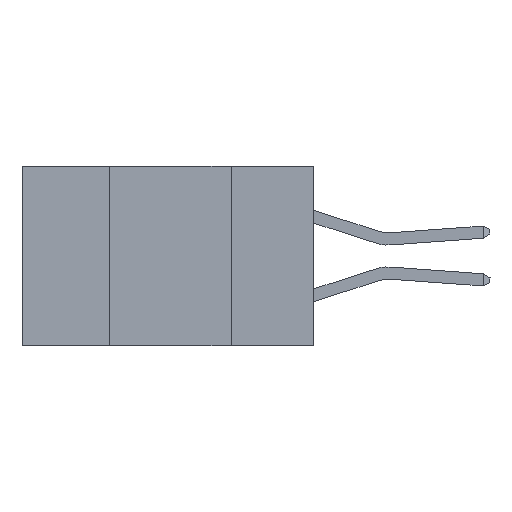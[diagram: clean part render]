
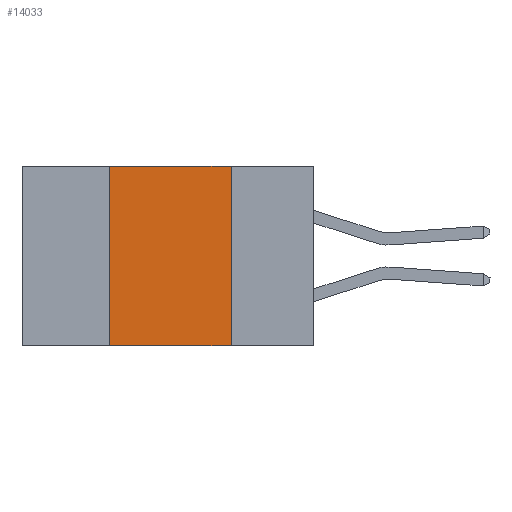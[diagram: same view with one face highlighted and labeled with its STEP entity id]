
A CAD part, left-side view. The second image highlights one B-rep face of the part: STEP entity #14033.
In plain terms, the highlighted planar face has unit normal (-1, 0, 0).
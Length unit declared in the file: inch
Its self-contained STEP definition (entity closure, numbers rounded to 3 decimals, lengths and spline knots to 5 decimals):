
#760 = CARTESIAN_POINT ( 'NONE',  ( 0., 0.17, 0. ) ) ;
#1239 = CARTESIAN_POINT ( 'NONE',  ( 0., 0.42, -0.37 ) ) ;
#2269 = VECTOR ( 'NONE', #9931, 39.37008 ) ;
#2905 = VECTOR ( 'NONE', #11522, 39.37008 ) ;
#3263 = CARTESIAN_POINT ( 'NONE',  ( 0., 0.6, -0.37 ) ) ;
#3797 = EDGE_CURVE ( 'NONE', #12333, #7902, #7656, .T. ) ;
#4444 = ORIENTED_EDGE ( 'NONE', *, *, #6841, .F. ) ;
#4681 = PLANE ( 'NONE',  #9546 ) ;
#4725 = LINE ( 'NONE', #14115, #2269 ) ;
#4855 = DIRECTION ( 'NONE',  ( 0., 0., -1. ) ) ;
#4933 = CARTESIAN_POINT ( 'NONE',  ( 0., 0.6, 0. ) ) ;
#5005 = VECTOR ( 'NONE', #7661, 39.37008 ) ;
#5102 = CARTESIAN_POINT ( 'NONE',  ( 0., 0.17, 0. ) ) ;
#5761 = ORIENTED_EDGE ( 'NONE', *, *, #12756, .F. ) ;
#6006 = ORIENTED_EDGE ( 'NONE', *, *, #17305, .F. ) ;
#6174 = DIRECTION ( 'NONE',  ( 1., 0., 0. ) ) ;
#6841 = EDGE_CURVE ( 'NONE', #12333, #11313, #11276, .T. ) ;
#7656 = LINE ( 'NONE', #3263, #2905 ) ;
#7661 = DIRECTION ( 'NONE',  ( 0., 0., -1. ) ) ;
#7736 = CARTESIAN_POINT ( 'NONE',  ( 0., 0.42, 0. ) ) ;
#7902 = VERTEX_POINT ( 'NONE', #9262 ) ;
#7913 = LINE ( 'NONE', #5102, #5005 ) ;
#8389 = FACE_OUTER_BOUND ( 'NONE', #14256, .T. ) ;
#9262 = CARTESIAN_POINT ( 'NONE',  ( 0., 0.17, -0.37 ) ) ;
#9546 = AXIS2_PLACEMENT_3D ( 'NONE', #4933, #6174, #4855 ) ;
#9931 = DIRECTION ( 'NONE',  ( 0., -1., 0. ) ) ;
#11276 = LINE ( 'NONE', #12757, #16647 ) ;
#11313 = VERTEX_POINT ( 'NONE', #7736 ) ;
#11522 = DIRECTION ( 'NONE',  ( 0., -1., 0. ) ) ;
#12333 = VERTEX_POINT ( 'NONE', #1239 ) ;
#12349 = ORIENTED_EDGE ( 'NONE', *, *, #3797, .T. ) ;
#12670 = DIRECTION ( 'NONE',  ( 0., 0., 1. ) ) ;
#12756 = EDGE_CURVE ( 'NONE', #14759, #7902, #7913, .T. ) ;
#12757 = CARTESIAN_POINT ( 'NONE',  ( 0., 0.42, 0. ) ) ;
#14033 = ADVANCED_FACE ( 'NONE', ( #8389 ), #4681, .F. ) ;
#14115 = CARTESIAN_POINT ( 'NONE',  ( 0., 0.6, 0. ) ) ;
#14256 = EDGE_LOOP ( 'NONE', ( #5761, #6006, #4444, #12349 ) ) ;
#14759 = VERTEX_POINT ( 'NONE', #760 ) ;
#16647 = VECTOR ( 'NONE', #12670, 39.37008 ) ;
#17305 = EDGE_CURVE ( 'NONE', #11313, #14759, #4725, .T. ) ;
